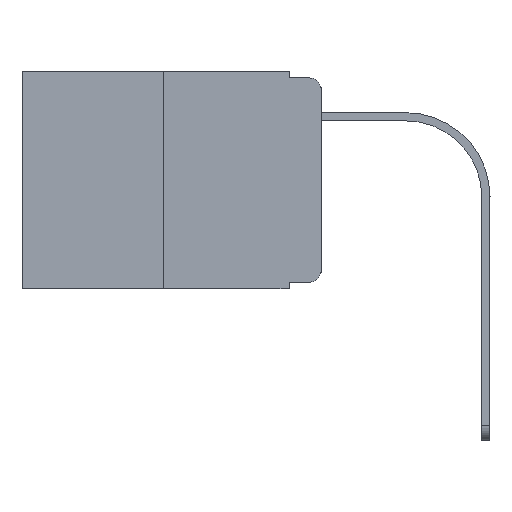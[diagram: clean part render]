
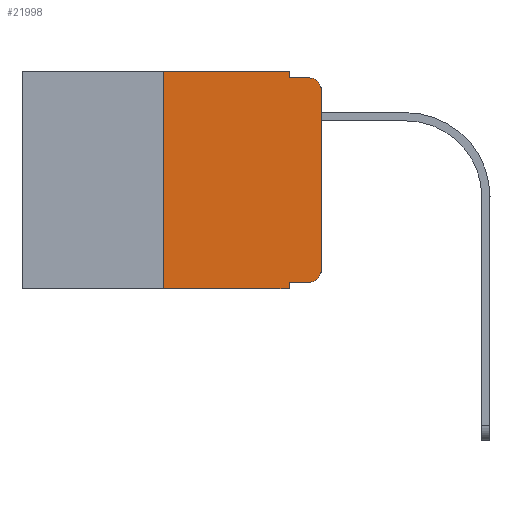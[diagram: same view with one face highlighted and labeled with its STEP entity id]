
A CAD part, left-side view. The second image highlights one B-rep face of the part: STEP entity #21998.
In plain terms, the highlighted planar face has unit normal (-1, 0, 0).
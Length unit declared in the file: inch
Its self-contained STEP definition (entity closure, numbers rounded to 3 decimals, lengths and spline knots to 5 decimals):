
#817 = LINE ( 'NONE', #1064, #14828 ) ;
#895 = EDGE_CURVE ( 'NONE', #19190, #16021, #20562, .T. ) ;
#1011 = PLANE ( 'NONE',  #14036 ) ;
#1064 = CARTESIAN_POINT ( 'NONE',  ( 0., 0.051, 0. ) ) ;
#1229 = ORIENTED_EDGE ( 'NONE', *, *, #2367, .F. ) ;
#1295 = LINE ( 'NONE', #23168, #13471 ) ;
#1299 = VECTOR ( 'NONE', #2818, 39.37008 ) ;
#2032 = ORIENTED_EDGE ( 'NONE', *, *, #19032, .F. ) ;
#2034 = CARTESIAN_POINT ( 'NONE',  ( 0., 0.02, -0.333 ) ) ;
#2367 = EDGE_CURVE ( 'NONE', #18307, #17558, #1295, .T. ) ;
#2483 = DIRECTION ( 'NONE',  ( 0., -1., 0. ) ) ;
#2818 = DIRECTION ( 'NONE',  ( 0., -1., 0. ) ) ;
#3008 = ORIENTED_EDGE ( 'NONE', *, *, #23448, .T. ) ;
#3359 = CARTESIAN_POINT ( 'NONE',  ( 0., 0.051, -0.343 ) ) ;
#5024 = CARTESIAN_POINT ( 'NONE',  ( 0., 0.25, 0. ) ) ;
#5247 = VECTOR ( 'NONE', #6980, 39.37008 ) ;
#5517 = VECTOR ( 'NONE', #2483, 39.37008 ) ;
#5991 = DIRECTION ( 'NONE',  ( 0., 0., -1. ) ) ;
#6226 = EDGE_CURVE ( 'NONE', #17558, #16021, #17542, .T. ) ;
#6658 = DIRECTION ( 'NONE',  ( 0., 0., -1. ) ) ;
#6980 = DIRECTION ( 'NONE',  ( 0., -1., 0. ) ) ;
#7394 = VERTEX_POINT ( 'NONE', #3359 ) ;
#7762 = DIRECTION ( 'NONE',  ( 0., 0., 1. ) ) ;
#8761 = LINE ( 'NONE', #19502, #1299 ) ;
#8848 = LINE ( 'NONE', #13241, #19069 ) ;
#8888 = CIRCLE ( 'NONE', #17162, 0.02 ) ;
#9527 = CARTESIAN_POINT ( 'NONE',  ( 0., 0.051, 0. ) ) ;
#9692 = CARTESIAN_POINT ( 'NONE',  ( 0., 0., -0.03 ) ) ;
#9855 = VECTOR ( 'NONE', #12301, 39.37008 ) ;
#10199 = CARTESIAN_POINT ( 'NONE',  ( 0., 0.473, -0.343 ) ) ;
#10400 = DIRECTION ( 'NONE',  ( 0., 0., -1. ) ) ;
#10578 = ORIENTED_EDGE ( 'NONE', *, *, #12732, .F. ) ;
#10804 = CARTESIAN_POINT ( 'NONE',  ( 0., 0.473, 0. ) ) ;
#10978 = ORIENTED_EDGE ( 'NONE', *, *, #895, .T. ) ;
#11005 = EDGE_CURVE ( 'NONE', #22329, #7394, #16017, .T. ) ;
#12301 = DIRECTION ( 'NONE',  ( 0., -1., 0. ) ) ;
#12489 = FACE_OUTER_BOUND ( 'NONE', #16013, .T. ) ;
#12644 = VERTEX_POINT ( 'NONE', #15754 ) ;
#12732 = EDGE_CURVE ( 'NONE', #22329, #15679, #8848, .T. ) ;
#13241 = CARTESIAN_POINT ( 'NONE',  ( 0., 0.25, 0. ) ) ;
#13471 = VECTOR ( 'NONE', #21468, 39.37008 ) ;
#13533 = EDGE_CURVE ( 'NONE', #19519, #19961, #8761, .T. ) ;
#13546 = CARTESIAN_POINT ( 'NONE',  ( 0., 0.02, -0.03 ) ) ;
#13731 = CARTESIAN_POINT ( 'NONE',  ( 0., 0.051, -0.01 ) ) ;
#13790 = DIRECTION ( 'NONE',  ( -1., 0., 0. ) ) ;
#14032 = CARTESIAN_POINT ( 'NONE',  ( 0., 0.051, -0.01 ) ) ;
#14036 = AXIS2_PLACEMENT_3D ( 'NONE', #16327, #17925, #10400 ) ;
#14221 = ORIENTED_EDGE ( 'NONE', *, *, #13533, .T. ) ;
#14415 = CARTESIAN_POINT ( 'NONE',  ( 0., 0.02, -0.01 ) ) ;
#14443 = CARTESIAN_POINT ( 'NONE',  ( 0., 0.02, -0.313 ) ) ;
#14801 = VECTOR ( 'NONE', #7762, 39.37008 ) ;
#14828 = VECTOR ( 'NONE', #21327, 39.37008 ) ;
#14885 = LINE ( 'NONE', #10804, #5247 ) ;
#14929 = LINE ( 'NONE', #20827, #14801 ) ;
#15326 = CARTESIAN_POINT ( 'NONE',  ( 0., 0.25, -0.343 ) ) ;
#15679 = VERTEX_POINT ( 'NONE', #5024 ) ;
#15754 = CARTESIAN_POINT ( 'NONE',  ( 0., 0., -0.313 ) ) ;
#16013 = EDGE_LOOP ( 'NONE', ( #21051, #10978, #17647, #1229, #2032, #10578, #22584, #17812, #14221, #3008 ) ) ;
#16017 = LINE ( 'NONE', #10199, #9855 ) ;
#16021 = VERTEX_POINT ( 'NONE', #14415 ) ;
#16327 = CARTESIAN_POINT ( 'NONE',  ( 0., 0.473, 0. ) ) ;
#16375 = DIRECTION ( 'NONE',  ( 0., 0., 1. ) ) ;
#17008 = AXIS2_PLACEMENT_3D ( 'NONE', #13546, #13790, #5991 ) ;
#17162 = AXIS2_PLACEMENT_3D ( 'NONE', #14443, #21950, #6658 ) ;
#17542 = LINE ( 'NONE', #13731, #5517 ) ;
#17558 = VERTEX_POINT ( 'NONE', #14032 ) ;
#17647 = ORIENTED_EDGE ( 'NONE', *, *, #6226, .F. ) ;
#17812 = ORIENTED_EDGE ( 'NONE', *, *, #23950, .F. ) ;
#17925 = DIRECTION ( 'NONE',  ( 1., 0., 0. ) ) ;
#18307 = VERTEX_POINT ( 'NONE', #9527 ) ;
#19032 = EDGE_CURVE ( 'NONE', #15679, #18307, #14885, .T. ) ;
#19069 = VECTOR ( 'NONE', #16375, 39.37008 ) ;
#19190 = VERTEX_POINT ( 'NONE', #9692 ) ;
#19502 = CARTESIAN_POINT ( 'NONE',  ( 0., 0.051, -0.333 ) ) ;
#19519 = VERTEX_POINT ( 'NONE', #22436 ) ;
#19615 = EDGE_CURVE ( 'NONE', #12644, #19190, #14929, .T. ) ;
#19961 = VERTEX_POINT ( 'NONE', #2034 ) ;
#20562 = CIRCLE ( 'NONE', #17008, 0.02 ) ;
#20827 = CARTESIAN_POINT ( 'NONE',  ( 0., 0., 0. ) ) ;
#21051 = ORIENTED_EDGE ( 'NONE', *, *, #19615, .T. ) ;
#21327 = DIRECTION ( 'NONE',  ( 0., 0., -1. ) ) ;
#21468 = DIRECTION ( 'NONE',  ( 0., 0., -1. ) ) ;
#21950 = DIRECTION ( 'NONE',  ( -1., 0., 0. ) ) ;
#21998 = ADVANCED_FACE ( 'NONE', ( #12489 ), #1011, .F. ) ;
#22329 = VERTEX_POINT ( 'NONE', #15326 ) ;
#22436 = CARTESIAN_POINT ( 'NONE',  ( 0., 0.051, -0.333 ) ) ;
#22584 = ORIENTED_EDGE ( 'NONE', *, *, #11005, .T. ) ;
#23168 = CARTESIAN_POINT ( 'NONE',  ( 0., 0.051, 0. ) ) ;
#23448 = EDGE_CURVE ( 'NONE', #19961, #12644, #8888, .T. ) ;
#23950 = EDGE_CURVE ( 'NONE', #19519, #7394, #817, .T. ) ;
